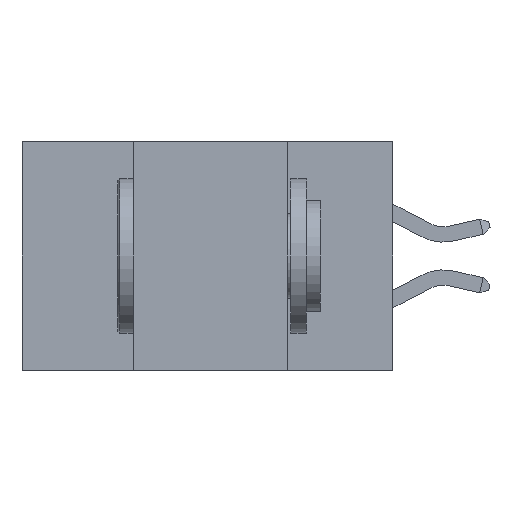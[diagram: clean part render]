
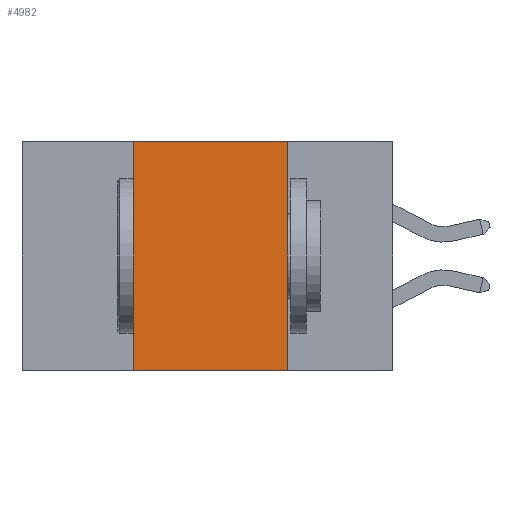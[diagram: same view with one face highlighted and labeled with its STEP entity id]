
A CAD part, left-side view. The second image highlights one B-rep face of the part: STEP entity #4982.
In plain terms, the highlighted planar face has unit normal (-1, 0, 0).
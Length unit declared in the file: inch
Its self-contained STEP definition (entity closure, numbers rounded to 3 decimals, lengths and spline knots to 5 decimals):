
#468 = LINE ( 'NONE', #786, #5592 ) ;
#786 = CARTESIAN_POINT ( 'NONE',  ( 0., 0.6, -0.37 ) ) ;
#967 = DIRECTION ( 'NONE',  ( 0., 0., -1. ) ) ;
#1007 = CARTESIAN_POINT ( 'NONE',  ( 0., 0.17, 0. ) ) ;
#1098 = CARTESIAN_POINT ( 'NONE',  ( 0., 0.42, -0.37 ) ) ;
#1277 = PLANE ( 'NONE',  #13138 ) ;
#1631 = CARTESIAN_POINT ( 'NONE',  ( 0., 0.17, 0. ) ) ;
#2828 = EDGE_CURVE ( 'NONE', #8585, #11551, #11185, .T. ) ;
#2837 = ORIENTED_EDGE ( 'NONE', *, *, #6782, .T. ) ;
#3048 = VECTOR ( 'NONE', #967, 39.37008 ) ;
#3474 = LINE ( 'NONE', #8852, #11309 ) ;
#3721 = EDGE_CURVE ( 'NONE', #6934, #10052, #5786, .T. ) ;
#3771 = DIRECTION ( 'NONE',  ( 0., 0., 1. ) ) ;
#3816 = CARTESIAN_POINT ( 'NONE',  ( 0., 0.42, 0. ) ) ;
#4538 = CARTESIAN_POINT ( 'NONE',  ( 0., 0.17, -0.37 ) ) ;
#4982 = ADVANCED_FACE ( 'NONE', ( #10879 ), #1277, .F. ) ;
#5158 = EDGE_CURVE ( 'NONE', #10052, #8585, #3474, .T. ) ;
#5592 = VECTOR ( 'NONE', #8940, 39.37008 ) ;
#5786 = LINE ( 'NONE', #3816, #8232 ) ;
#6782 = EDGE_CURVE ( 'NONE', #6934, #11551, #468, .T. ) ;
#6830 = ORIENTED_EDGE ( 'NONE', *, *, #5158, .F. ) ;
#6934 = VERTEX_POINT ( 'NONE', #1098 ) ;
#7172 = ORIENTED_EDGE ( 'NONE', *, *, #3721, .F. ) ;
#7590 = DIRECTION ( 'NONE',  ( 1., 0., 0. ) ) ;
#7603 = DIRECTION ( 'NONE',  ( 0., 0., -1. ) ) ;
#7618 = CARTESIAN_POINT ( 'NONE',  ( 0., 0.6, 0. ) ) ;
#8093 = DIRECTION ( 'NONE',  ( 0., -1., 0. ) ) ;
#8232 = VECTOR ( 'NONE', #3771, 39.37008 ) ;
#8585 = VERTEX_POINT ( 'NONE', #1631 ) ;
#8852 = CARTESIAN_POINT ( 'NONE',  ( 0., 0.6, 0. ) ) ;
#8940 = DIRECTION ( 'NONE',  ( 0., -1., 0. ) ) ;
#9106 = ORIENTED_EDGE ( 'NONE', *, *, #2828, .F. ) ;
#9881 = EDGE_LOOP ( 'NONE', ( #9106, #6830, #7172, #2837 ) ) ;
#10052 = VERTEX_POINT ( 'NONE', #10489 ) ;
#10489 = CARTESIAN_POINT ( 'NONE',  ( 0., 0.42, 0. ) ) ;
#10879 = FACE_OUTER_BOUND ( 'NONE', #9881, .T. ) ;
#11185 = LINE ( 'NONE', #1007, #3048 ) ;
#11309 = VECTOR ( 'NONE', #8093, 39.37008 ) ;
#11551 = VERTEX_POINT ( 'NONE', #4538 ) ;
#13138 = AXIS2_PLACEMENT_3D ( 'NONE', #7618, #7590, #7603 ) ;
